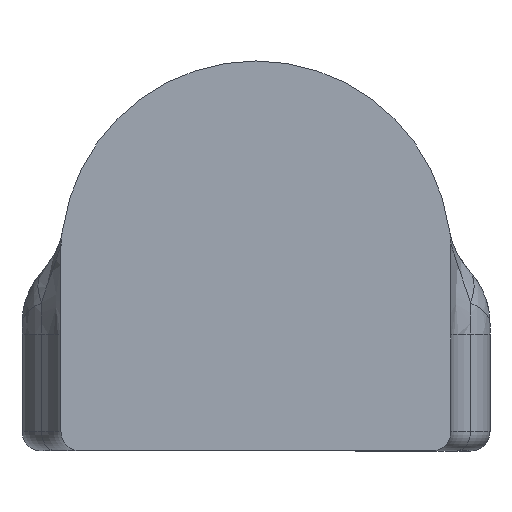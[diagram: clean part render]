
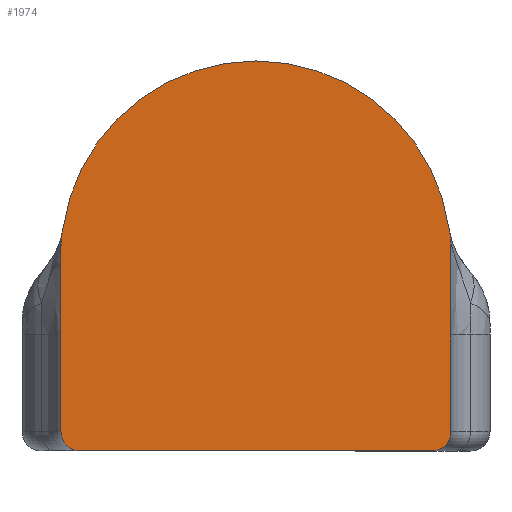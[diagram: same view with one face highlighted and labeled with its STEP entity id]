
A CAD part, left-side view. The second image highlights one B-rep face of the part: STEP entity #1974.
In plain terms, the highlighted planar face has unit normal (-1, 0, 0).
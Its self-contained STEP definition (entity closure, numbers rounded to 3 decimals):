
#35 = DIRECTION ( 'NONE',  ( 1., 0., 0. ) ) ;
#36 = CARTESIAN_POINT ( 'NONE',  ( 0., 2.5, -2.25 ) ) ;
#55 = EDGE_CURVE ( 'NONE', #2190, #332, #233, .T. ) ;
#66 = CARTESIAN_POINT ( 'NONE',  ( 0., 2.25, -2.25 ) ) ;
#72 = DIRECTION ( 'NONE',  ( 0., 0., -1. ) ) ;
#119 = ORIENTED_EDGE ( 'NONE', *, *, #1801, .T. ) ;
#137 = CARTESIAN_POINT ( 'NONE',  ( 0., 2.482, 0.309 ) ) ;
#145 = DIRECTION ( 'NONE',  ( 1., 0., 0. ) ) ;
#155 = AXIS2_PLACEMENT_3D ( 'NONE', #1057, #35, #1238 ) ;
#190 = CARTESIAN_POINT ( 'NONE',  ( 0., -2.475, 0.354 ) ) ;
#195 = AXIS2_PLACEMENT_3D ( 'NONE', #420, #1651, #598 ) ;
#198 = CARTESIAN_POINT ( 'NONE',  ( 0., -2.25, -2.5 ) ) ;
#221 = ORIENTED_EDGE ( 'NONE', *, *, #798, .T. ) ;
#233 = CIRCLE ( 'NONE', #1869, 1. ) ;
#235 = EDGE_CURVE ( 'NONE', #783, #568, #1340, .T. ) ;
#242 = DIRECTION ( 'NONE',  ( 0., 0., -1. ) ) ;
#265 = CIRCLE ( 'NONE', #1201, 0.25 ) ;
#282 = ORIENTED_EDGE ( 'NONE', *, *, #1754, .F. ) ;
#329 = VECTOR ( 'NONE', #596, 1000. ) ;
#332 = VERTEX_POINT ( 'NONE', #2118 ) ;
#337 = CIRCLE ( 'NONE', #440, 2.5 ) ;
#352 = DIRECTION ( 'NONE',  ( 1., 0., 0. ) ) ;
#360 = ORIENTED_EDGE ( 'NONE', *, *, #55, .T. ) ;
#419 = LINE ( 'NONE', #1040, #1279 ) ;
#420 = CARTESIAN_POINT ( 'NONE',  ( 0., -2.25, -2.25 ) ) ;
#424 = CIRCLE ( 'NONE', #1731, 1. ) ;
#440 = AXIS2_PLACEMENT_3D ( 'NONE', #1697, #633, #1880 ) ;
#444 = EDGE_LOOP ( 'NONE', ( #119, #221, #282, #360, #677, #729, #882, #956, #1017, #1109, #1220 ) ) ;
#536 = VERTEX_POINT ( 'NONE', #1324 ) ;
#568 = VERTEX_POINT ( 'NONE', #2244 ) ;
#587 = CIRCLE ( 'NONE', #195, 0.25 ) ;
#590 = CARTESIAN_POINT ( 'NONE',  ( 0., 2.475, 0.354 ) ) ;
#596 = DIRECTION ( 'NONE',  ( 0., 0., -1. ) ) ;
#598 = DIRECTION ( 'NONE',  ( 0., 0., -1. ) ) ;
#610 = DIRECTION ( 'NONE',  ( 0., -1., 0. ) ) ;
#625 = EDGE_CURVE ( 'NONE', #568, #984, #337, .T. ) ;
#633 = DIRECTION ( 'NONE',  ( 1., 0., 0. ) ) ;
#676 = VERTEX_POINT ( 'NONE', #2077 ) ;
#677 = ORIENTED_EDGE ( 'NONE', *, *, #1741, .T. ) ;
#729 = ORIENTED_EDGE ( 'NONE', *, *, #625, .F. ) ;
#760 = DIRECTION ( 'NONE',  ( 1., 0., 0. ) ) ;
#783 = VERTEX_POINT ( 'NONE', #590 ) ;
#794 = VERTEX_POINT ( 'NONE', #1087 ) ;
#798 = EDGE_CURVE ( 'NONE', #2157, #794, #587, .T. ) ;
#857 = EDGE_CURVE ( 'NONE', #1906, #676, #424, .T. ) ;
#858 = PLANE ( 'NONE',  #1672 ) ;
#882 = ORIENTED_EDGE ( 'NONE', *, *, #235, .F. ) ;
#950 = AXIS2_PLACEMENT_3D ( 'NONE', #1166, #145, #1351 ) ;
#956 = ORIENTED_EDGE ( 'NONE', *, *, #996, .T. ) ;
#984 = VERTEX_POINT ( 'NONE', #190 ) ;
#996 = EDGE_CURVE ( 'NONE', #783, #1906, #1110, .T. ) ;
#1017 = ORIENTED_EDGE ( 'NONE', *, *, #857, .T. ) ;
#1029 = CARTESIAN_POINT ( 'NONE',  ( 0., 0., 0. ) ) ;
#1040 = CARTESIAN_POINT ( 'NONE',  ( 0., 2.5, 0. ) ) ;
#1053 = DIRECTION ( 'NONE',  ( 0., 0., -1. ) ) ;
#1057 = CARTESIAN_POINT ( 'NONE',  ( 0., 3.465, 0.496 ) ) ;
#1066 = DIRECTION ( 'NONE',  ( -1., 0., 0. ) ) ;
#1087 = CARTESIAN_POINT ( 'NONE',  ( 0., -2.5, -2.25 ) ) ;
#1090 = DIRECTION ( 'NONE',  ( -1., 0., 0. ) ) ;
#1092 = CARTESIAN_POINT ( 'NONE',  ( 0., -1.5, 0.122 ) ) ;
#1109 = ORIENTED_EDGE ( 'NONE', *, *, #2052, .T. ) ;
#1110 = CIRCLE ( 'NONE', #155, 1. ) ;
#1119 = EDGE_CURVE ( 'NONE', #2112, #536, #265, .T. ) ;
#1130 = LINE ( 'NONE', #1851, #2061 ) ;
#1166 = CARTESIAN_POINT ( 'NONE',  ( 0., 0., 0. ) ) ;
#1201 = AXIS2_PLACEMENT_3D ( 'NONE', #66, #1271, #242 ) ;
#1210 = AXIS2_PLACEMENT_3D ( 'NONE', #1839, #760, #2021 ) ;
#1220 = ORIENTED_EDGE ( 'NONE', *, *, #1119, .T. ) ;
#1226 = DIRECTION ( 'NONE',  ( 0., 0., -1. ) ) ;
#1238 = DIRECTION ( 'NONE',  ( 0., 0., -1. ) ) ;
#1271 = DIRECTION ( 'NONE',  ( -1., 0., 0. ) ) ;
#1279 = VECTOR ( 'NONE', #1226, 1000. ) ;
#1307 = LINE ( 'NONE', #1647, #329 ) ;
#1324 = CARTESIAN_POINT ( 'NONE',  ( 0., 2.25, -2.5 ) ) ;
#1340 = CIRCLE ( 'NONE', #950, 2.5 ) ;
#1351 = DIRECTION ( 'NONE',  ( 0., 0., -1. ) ) ;
#1456 = FACE_OUTER_BOUND ( 'NONE', #444, .T. ) ;
#1584 = DIRECTION ( 'NONE',  ( 0., 0., -1. ) ) ;
#1604 = CARTESIAN_POINT ( 'NONE',  ( 0., -2.5, 0.122 ) ) ;
#1647 = CARTESIAN_POINT ( 'NONE',  ( 0., -2.5, 0. ) ) ;
#1651 = DIRECTION ( 'NONE',  ( -1., 0., 0. ) ) ;
#1672 = AXIS2_PLACEMENT_3D ( 'NONE', #1029, #352, #1584 ) ;
#1697 = CARTESIAN_POINT ( 'NONE',  ( 0., 0., 0. ) ) ;
#1731 = AXIS2_PLACEMENT_3D ( 'NONE', #2195, #1090, #72 ) ;
#1741 = EDGE_CURVE ( 'NONE', #332, #984, #2224, .T. ) ;
#1754 = EDGE_CURVE ( 'NONE', #2190, #794, #1307, .T. ) ;
#1801 = EDGE_CURVE ( 'NONE', #536, #2157, #1130, .T. ) ;
#1839 = CARTESIAN_POINT ( 'NONE',  ( 0., -3.465, 0.496 ) ) ;
#1851 = CARTESIAN_POINT ( 'NONE',  ( 0., 0., -2.5 ) ) ;
#1869 = AXIS2_PLACEMENT_3D ( 'NONE', #1092, #1066, #1053 ) ;
#1880 = DIRECTION ( 'NONE',  ( 0., 0., -1. ) ) ;
#1906 = VERTEX_POINT ( 'NONE', #137 ) ;
#1974 = ADVANCED_FACE ( 'NONE', ( #1456 ), #858, .F. ) ;
#2021 = DIRECTION ( 'NONE',  ( 0., 0., -1. ) ) ;
#2052 = EDGE_CURVE ( 'NONE', #676, #2112, #419, .T. ) ;
#2061 = VECTOR ( 'NONE', #610, 1000. ) ;
#2077 = CARTESIAN_POINT ( 'NONE',  ( 0., 2.5, 0.122 ) ) ;
#2112 = VERTEX_POINT ( 'NONE', #36 ) ;
#2118 = CARTESIAN_POINT ( 'NONE',  ( 0., -2.482, 0.309 ) ) ;
#2157 = VERTEX_POINT ( 'NONE', #198 ) ;
#2190 = VERTEX_POINT ( 'NONE', #1604 ) ;
#2195 = CARTESIAN_POINT ( 'NONE',  ( 0., 1.5, 0.122 ) ) ;
#2224 = CIRCLE ( 'NONE', #1210, 1. ) ;
#2244 = CARTESIAN_POINT ( 'NONE',  ( 0., 0., 2.5 ) ) ;
